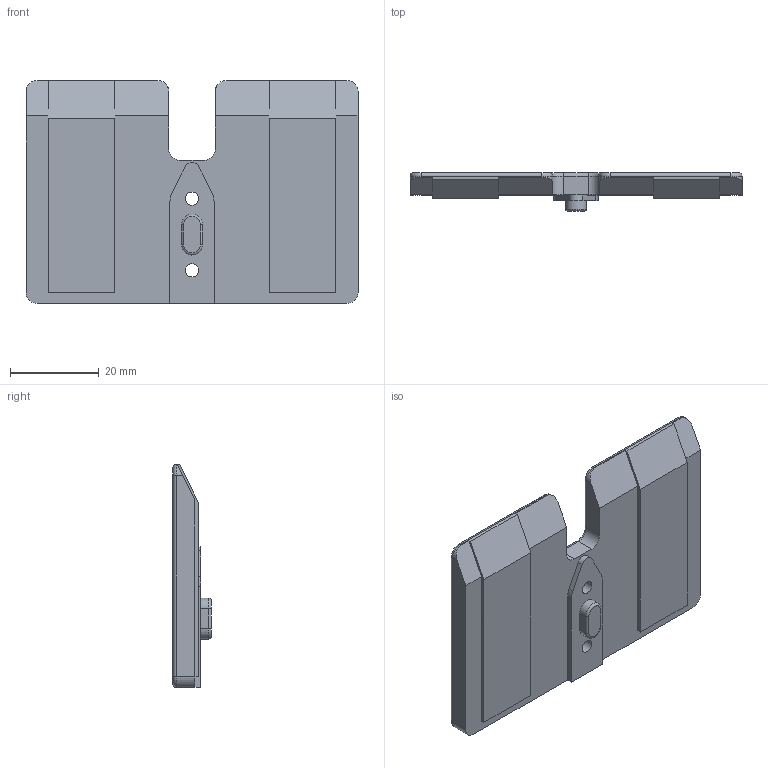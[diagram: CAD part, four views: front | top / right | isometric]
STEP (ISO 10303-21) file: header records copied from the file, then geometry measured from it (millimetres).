
FILE_DESCRIPTION(/* description */ (''),/* implementation_level */ '2;1');
FILE_NAME(/* name */ 'Glock 17 mag holder v19.step',/* time_stamp */ '2022-02-11T12:47:34-05:00',/* author */ (''),/* organization */ (''),/* preprocessor_version */ 'ST-DEVELOPER v18.1',/* originating_system */ 'Autodesk Translation Framework v10.13.0.1454',/* authorisation */ '');
FILE_SCHEMA (('AUTOMOTIVE_DESIGN { 1 0 10303 214 3 1 1 }'));
Length unit declared in the file: millimetre
Products named in the file (1): Glock 17 mag holder
Bounding box: 75 x 8.65 x 50.37 mm (x, y, z)
Volume: 18111.5 mm3; surface area: 8759.6 mm2
Topology: 1 solids, 1 shells, 155 faces, 406 edges, 264 vertices
Faces by surface type: plane 86, cylinder 35, bspline 22, torus 12
Full cylindrical faces by diameter (mm): 3 x2, 5.75 x2
Entity records: 4833 total; most frequent: CARTESIAN_POINT 1112, ORIENTED_EDGE 812, DIRECTION 716, EDGE_CURVE 406, LINE 276, VECTOR 276, VERTEX_POINT 264, AXIS2_PLACEMENT_3D 220
